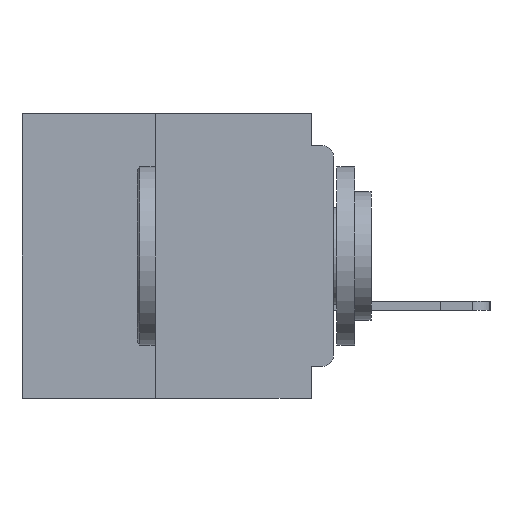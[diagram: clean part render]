
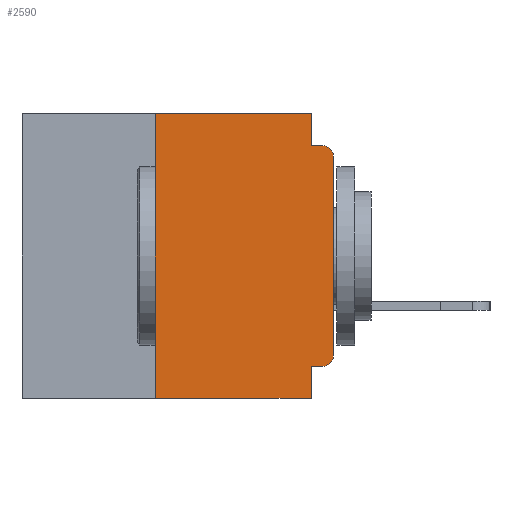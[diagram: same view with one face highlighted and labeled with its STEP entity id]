
A CAD part, left-side view. The second image highlights one B-rep face of the part: STEP entity #2590.
In plain terms, the highlighted planar face has unit normal (-1, 0, 0).
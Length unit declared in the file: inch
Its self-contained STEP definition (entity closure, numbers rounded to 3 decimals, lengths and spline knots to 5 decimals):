
#150 = CARTESIAN_POINT ( 'NONE',  ( 0., 0., 0. ) ) ;
#1692 = CARTESIAN_POINT ( 'NONE',  ( 0., 0.25, 0. ) ) ;
#2425 = CARTESIAN_POINT ( 'NONE',  ( 0., 0., -0.045 ) ) ;
#2526 = DIRECTION ( 'NONE',  ( 0., 0., -1. ) ) ;
#2590 = ADVANCED_FACE ( 'NONE', ( #23719 ), #26259, .F. ) ;
#3111 = CARTESIAN_POINT ( 'NONE',  ( 0., 0.031, -0.355 ) ) ;
#3409 = VECTOR ( 'NONE', #34255, 39.37008 ) ;
#4150 = EDGE_CURVE ( 'NONE', #58841, #24554, #53278, .T. ) ;
#4334 = VECTOR ( 'NONE', #16334, 39.37008 ) ;
#4904 = CARTESIAN_POINT ( 'NONE',  ( 0., 0.031, 0. ) ) ;
#5727 = DIRECTION ( 'NONE',  ( -1., 0., 0. ) ) ;
#5807 = CARTESIAN_POINT ( 'NONE',  ( 0., 0.25, -0.4 ) ) ;
#6336 = EDGE_CURVE ( 'NONE', #12257, #47325, #33284, .T. ) ;
#6945 = CARTESIAN_POINT ( 'NONE',  ( 0., 0.031, -0.4 ) ) ;
#6996 = ORIENTED_EDGE ( 'NONE', *, *, #41714, .T. ) ;
#7176 = DIRECTION ( 'NONE',  ( 0., -1., 0. ) ) ;
#8319 = VERTEX_POINT ( 'NONE', #37420 ) ;
#10273 = ORIENTED_EDGE ( 'NONE', *, *, #28503, .F. ) ;
#11156 = EDGE_CURVE ( 'NONE', #47325, #45122, #45410, .T. ) ;
#12257 = VERTEX_POINT ( 'NONE', #59858 ) ;
#12435 = VECTOR ( 'NONE', #33354, 39.37008 ) ;
#12684 = ORIENTED_EDGE ( 'NONE', *, *, #19432, .F. ) ;
#13926 = LINE ( 'NONE', #150, #12435 ) ;
#14190 = CARTESIAN_POINT ( 'NONE',  ( 0., 0., -0.34 ) ) ;
#15439 = VERTEX_POINT ( 'NONE', #4904 ) ;
#16334 = DIRECTION ( 'NONE',  ( 0., -1., 0. ) ) ;
#16905 = CARTESIAN_POINT ( 'NONE',  ( 0., 0.437, 0. ) ) ;
#19432 = EDGE_CURVE ( 'NONE', #15439, #58841, #40712, .T. ) ;
#20242 = CIRCLE ( 'NONE', #43793, 0.015 ) ;
#20334 = VECTOR ( 'NONE', #58516, 39.37008 ) ;
#20627 = VECTOR ( 'NONE', #57506, 39.37008 ) ;
#21258 = CARTESIAN_POINT ( 'NONE',  ( 0., 0.015, -0.045 ) ) ;
#23379 = ORIENTED_EDGE ( 'NONE', *, *, #4150, .F. ) ;
#23719 = FACE_OUTER_BOUND ( 'NONE', #31516, .T. ) ;
#24554 = VERTEX_POINT ( 'NONE', #21258 ) ;
#24889 = CARTESIAN_POINT ( 'NONE',  ( 0., 0.437, -0.4 ) ) ;
#25853 = DIRECTION ( 'NONE',  ( 0., 0., -1. ) ) ;
#26179 = DIRECTION ( 'NONE',  ( 1., 0., 0. ) ) ;
#26259 = PLANE ( 'NONE',  #35531 ) ;
#28411 = VECTOR ( 'NONE', #7176, 39.37008 ) ;
#28503 = EDGE_CURVE ( 'NONE', #37044, #15439, #43536, .T. ) ;
#29861 = CARTESIAN_POINT ( 'NONE',  ( 0., 0., -0.06 ) ) ;
#30963 = DIRECTION ( 'NONE',  ( -1., 0., 0. ) ) ;
#31516 = EDGE_LOOP ( 'NONE', ( #45147, #43165, #23379, #12684, #10273, #41813, #48253, #38516, #49362, #6996 ) ) ;
#33284 = LINE ( 'NONE', #34118, #20627 ) ;
#33354 = DIRECTION ( 'NONE',  ( 0., 0., 1. ) ) ;
#33948 = DIRECTION ( 'NONE',  ( 0., 0., -1. ) ) ;
#34118 = CARTESIAN_POINT ( 'NONE',  ( 0., 0., -0.355 ) ) ;
#34176 = CARTESIAN_POINT ( 'NONE',  ( 0., 0.015, -0.06 ) ) ;
#34255 = DIRECTION ( 'NONE',  ( 0., 0., 1. ) ) ;
#35531 = AXIS2_PLACEMENT_3D ( 'NONE', #16905, #26179, #25853 ) ;
#36387 = AXIS2_PLACEMENT_3D ( 'NONE', #58850, #30963, #2526 ) ;
#37044 = VERTEX_POINT ( 'NONE', #1692 ) ;
#37420 = CARTESIAN_POINT ( 'NONE',  ( 0., 0.25, -0.4 ) ) ;
#37751 = CARTESIAN_POINT ( 'NONE',  ( 0., 0.031, -0.4 ) ) ;
#38253 = LINE ( 'NONE', #5807, #3409 ) ;
#38516 = ORIENTED_EDGE ( 'NONE', *, *, #11156, .F. ) ;
#38653 = CARTESIAN_POINT ( 'NONE',  ( 0., 0.031, 0. ) ) ;
#38863 = DIRECTION ( 'NONE',  ( 0., 0., -1. ) ) ;
#39594 = VERTEX_POINT ( 'NONE', #14190 ) ;
#40712 = LINE ( 'NONE', #38653, #51660 ) ;
#41714 = EDGE_CURVE ( 'NONE', #12257, #39594, #54585, .T. ) ;
#41813 = ORIENTED_EDGE ( 'NONE', *, *, #58514, .F. ) ;
#43165 = ORIENTED_EDGE ( 'NONE', *, *, #49344, .T. ) ;
#43493 = EDGE_CURVE ( 'NONE', #8319, #45122, #59420, .T. ) ;
#43536 = LINE ( 'NONE', #49307, #4334 ) ;
#43793 = AXIS2_PLACEMENT_3D ( 'NONE', #34176, #5727, #38863 ) ;
#45122 = VERTEX_POINT ( 'NONE', #37751 ) ;
#45147 = ORIENTED_EDGE ( 'NONE', *, *, #45760, .T. ) ;
#45410 = LINE ( 'NONE', #6945, #20334 ) ;
#45760 = EDGE_CURVE ( 'NONE', #39594, #55965, #13926, .T. ) ;
#47325 = VERTEX_POINT ( 'NONE', #3111 ) ;
#48253 = ORIENTED_EDGE ( 'NONE', *, *, #43493, .T. ) ;
#48565 = VECTOR ( 'NONE', #57624, 39.37008 ) ;
#49307 = CARTESIAN_POINT ( 'NONE',  ( 0., 0.437, 0. ) ) ;
#49344 = EDGE_CURVE ( 'NONE', #55965, #24554, #20242, .T. ) ;
#49362 = ORIENTED_EDGE ( 'NONE', *, *, #6336, .F. ) ;
#51660 = VECTOR ( 'NONE', #33948, 39.37008 ) ;
#53278 = LINE ( 'NONE', #2425, #28411 ) ;
#54585 = CIRCLE ( 'NONE', #36387, 0.015 ) ;
#55564 = CARTESIAN_POINT ( 'NONE',  ( 0., 0.031, -0.045 ) ) ;
#55965 = VERTEX_POINT ( 'NONE', #29861 ) ;
#57506 = DIRECTION ( 'NONE',  ( 0., 1., 0. ) ) ;
#57624 = DIRECTION ( 'NONE',  ( 0., -1., 0. ) ) ;
#58514 = EDGE_CURVE ( 'NONE', #8319, #37044, #38253, .T. ) ;
#58516 = DIRECTION ( 'NONE',  ( 0., 0., -1. ) ) ;
#58841 = VERTEX_POINT ( 'NONE', #55564 ) ;
#58850 = CARTESIAN_POINT ( 'NONE',  ( 0., 0.015, -0.34 ) ) ;
#59420 = LINE ( 'NONE', #24889, #48565 ) ;
#59858 = CARTESIAN_POINT ( 'NONE',  ( 0., 0.015, -0.355 ) ) ;
